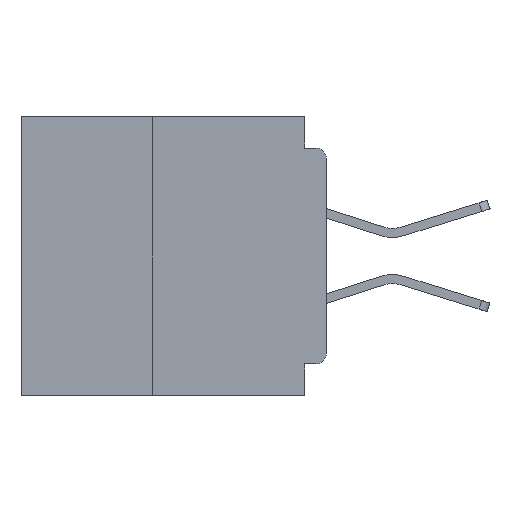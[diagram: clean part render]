
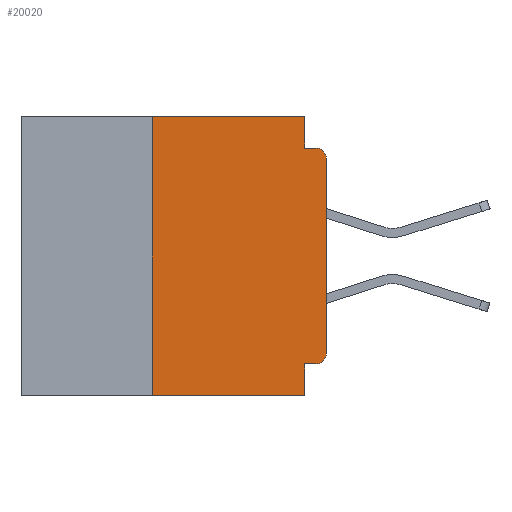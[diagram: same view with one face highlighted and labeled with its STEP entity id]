
A CAD part, left-side view. The second image highlights one B-rep face of the part: STEP entity #20020.
In plain terms, the highlighted planar face has unit normal (-1, 0, 0).
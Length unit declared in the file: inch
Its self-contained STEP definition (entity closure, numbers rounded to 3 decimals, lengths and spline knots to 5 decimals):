
#485 = VERTEX_POINT ( 'NONE', #10741 ) ;
#1508 = VERTEX_POINT ( 'NONE', #22685 ) ;
#1844 = EDGE_CURVE ( 'NONE', #33333, #43503, #17611, .T. ) ;
#2276 = LINE ( 'NONE', #12551, #21731 ) ;
#2382 = DIRECTION ( 'NONE',  ( 0., 0., -1. ) ) ;
#2426 = DIRECTION ( 'NONE',  ( -1., 0., 0. ) ) ;
#2542 = CARTESIAN_POINT ( 'NONE',  ( 0., 0.015, -0.34 ) ) ;
#2708 = CARTESIAN_POINT ( 'NONE',  ( 0., 0.25, -0.4 ) ) ;
#3090 = CARTESIAN_POINT ( 'NONE',  ( 0., 0.015, -0.06 ) ) ;
#3274 = ORIENTED_EDGE ( 'NONE', *, *, #20890, .T. ) ;
#4044 = VECTOR ( 'NONE', #33623, 39.37008 ) ;
#4313 = VECTOR ( 'NONE', #13646, 39.37008 ) ;
#4979 = ORIENTED_EDGE ( 'NONE', *, *, #45223, .T. ) ;
#5046 = CARTESIAN_POINT ( 'NONE',  ( 0., 0., 0. ) ) ;
#5235 = CARTESIAN_POINT ( 'NONE',  ( 0., 0.031, -0.4 ) ) ;
#6185 = ORIENTED_EDGE ( 'NONE', *, *, #1844, .T. ) ;
#6187 = CARTESIAN_POINT ( 'NONE',  ( 0., 0.031, 0. ) ) ;
#6771 = DIRECTION ( 'NONE',  ( 0., 0., -1. ) ) ;
#7290 = ORIENTED_EDGE ( 'NONE', *, *, #33402, .F. ) ;
#8015 = LINE ( 'NONE', #17584, #15412 ) ;
#8559 = CARTESIAN_POINT ( 'NONE',  ( 0., 0., -0.06 ) ) ;
#9506 = VECTOR ( 'NONE', #35073, 39.37008 ) ;
#10741 = CARTESIAN_POINT ( 'NONE',  ( 0., 0.25, 0. ) ) ;
#12551 = CARTESIAN_POINT ( 'NONE',  ( 0., 0.25, -0.4 ) ) ;
#12981 = ORIENTED_EDGE ( 'NONE', *, *, #31363, .F. ) ;
#13646 = DIRECTION ( 'NONE',  ( 0., -1., 0. ) ) ;
#14060 = EDGE_CURVE ( 'NONE', #43916, #42410, #25183, .T. ) ;
#14348 = EDGE_CURVE ( 'NONE', #485, #17065, #36266, .T. ) ;
#14482 = FACE_OUTER_BOUND ( 'NONE', #16953, .T. ) ;
#15412 = VECTOR ( 'NONE', #46090, 39.37008 ) ;
#16256 = DIRECTION ( 'NONE',  ( 0., 0., 1. ) ) ;
#16738 = VECTOR ( 'NONE', #22337, 39.37008 ) ;
#16953 = EDGE_LOOP ( 'NONE', ( #4979, #34946, #44351, #7290, #37173, #46570, #3274, #12981, #33877, #6185 ) ) ;
#17065 = VERTEX_POINT ( 'NONE', #38707 ) ;
#17584 = CARTESIAN_POINT ( 'NONE',  ( 0., 0., -0.355 ) ) ;
#17611 = CIRCLE ( 'NONE', #39202, 0.015 ) ;
#19466 = LINE ( 'NONE', #23106, #37329 ) ;
#20020 = ADVANCED_FACE ( 'NONE', ( #14482 ), #31617, .F. ) ;
#20890 = EDGE_CURVE ( 'NONE', #34475, #24712, #45187, .T. ) ;
#21149 = DIRECTION ( 'NONE',  ( 1., 0., 0. ) ) ;
#21731 = VECTOR ( 'NONE', #16256, 39.37008 ) ;
#22337 = DIRECTION ( 'NONE',  ( 0., -1., 0. ) ) ;
#22685 = CARTESIAN_POINT ( 'NONE',  ( 0., 0.031, -0.045 ) ) ;
#22843 = VECTOR ( 'NONE', #23404, 39.37008 ) ;
#23106 = CARTESIAN_POINT ( 'NONE',  ( 0., 0.031, -0.4 ) ) ;
#23404 = DIRECTION ( 'NONE',  ( 0., 0., 1. ) ) ;
#24712 = VERTEX_POINT ( 'NONE', #5235 ) ;
#25183 = CIRCLE ( 'NONE', #46369, 0.015 ) ;
#26548 = LINE ( 'NONE', #6187, #9506 ) ;
#26730 = DIRECTION ( 'NONE',  ( 0., 0., -1. ) ) ;
#28545 = DIRECTION ( 'NONE',  ( -1., 0., 0. ) ) ;
#29395 = CARTESIAN_POINT ( 'NONE',  ( 0., 0.437, -0.4 ) ) ;
#29396 = AXIS2_PLACEMENT_3D ( 'NONE', #42452, #21149, #45998 ) ;
#30053 = CARTESIAN_POINT ( 'NONE',  ( 0., 0.437, 0. ) ) ;
#31021 = EDGE_CURVE ( 'NONE', #33333, #40137, #8015, .T. ) ;
#31363 = EDGE_CURVE ( 'NONE', #40137, #24712, #19466, .T. ) ;
#31617 = PLANE ( 'NONE',  #29396 ) ;
#31677 = CARTESIAN_POINT ( 'NONE',  ( 0., 0.015, -0.045 ) ) ;
#33196 = LINE ( 'NONE', #42339, #4313 ) ;
#33333 = VERTEX_POINT ( 'NONE', #41729 ) ;
#33402 = EDGE_CURVE ( 'NONE', #17065, #1508, #26548, .T. ) ;
#33623 = DIRECTION ( 'NONE',  ( 0., -1., 0. ) ) ;
#33877 = ORIENTED_EDGE ( 'NONE', *, *, #31021, .F. ) ;
#34475 = VERTEX_POINT ( 'NONE', #2708 ) ;
#34946 = ORIENTED_EDGE ( 'NONE', *, *, #14060, .T. ) ;
#35073 = DIRECTION ( 'NONE',  ( 0., 0., -1. ) ) ;
#35584 = CARTESIAN_POINT ( 'NONE',  ( 0., 0.031, -0.355 ) ) ;
#36266 = LINE ( 'NONE', #30053, #4044 ) ;
#37173 = ORIENTED_EDGE ( 'NONE', *, *, #14348, .F. ) ;
#37329 = VECTOR ( 'NONE', #26730, 39.37008 ) ;
#37604 = EDGE_CURVE ( 'NONE', #1508, #42410, #33196, .T. ) ;
#37998 = CARTESIAN_POINT ( 'NONE',  ( 0., 0., -0.34 ) ) ;
#38707 = CARTESIAN_POINT ( 'NONE',  ( 0., 0.031, 0. ) ) ;
#39202 = AXIS2_PLACEMENT_3D ( 'NONE', #2542, #2426, #2382 ) ;
#40137 = VERTEX_POINT ( 'NONE', #35584 ) ;
#40623 = LINE ( 'NONE', #5046, #22843 ) ;
#41729 = CARTESIAN_POINT ( 'NONE',  ( 0., 0.015, -0.355 ) ) ;
#42339 = CARTESIAN_POINT ( 'NONE',  ( 0., 0., -0.045 ) ) ;
#42410 = VERTEX_POINT ( 'NONE', #31677 ) ;
#42452 = CARTESIAN_POINT ( 'NONE',  ( 0., 0.437, 0. ) ) ;
#43503 = VERTEX_POINT ( 'NONE', #37998 ) ;
#43916 = VERTEX_POINT ( 'NONE', #8559 ) ;
#44351 = ORIENTED_EDGE ( 'NONE', *, *, #37604, .F. ) ;
#45187 = LINE ( 'NONE', #29395, #16738 ) ;
#45223 = EDGE_CURVE ( 'NONE', #43503, #43916, #40623, .T. ) ;
#45248 = EDGE_CURVE ( 'NONE', #34475, #485, #2276, .T. ) ;
#45998 = DIRECTION ( 'NONE',  ( 0., 0., -1. ) ) ;
#46090 = DIRECTION ( 'NONE',  ( 0., 1., 0. ) ) ;
#46369 = AXIS2_PLACEMENT_3D ( 'NONE', #3090, #28545, #6771 ) ;
#46570 = ORIENTED_EDGE ( 'NONE', *, *, #45248, .F. ) ;
